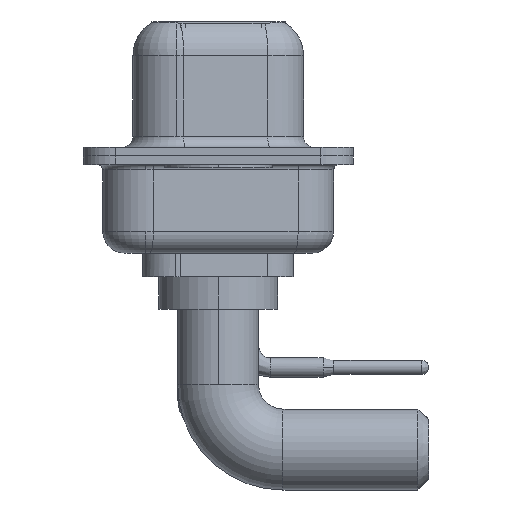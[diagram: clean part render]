
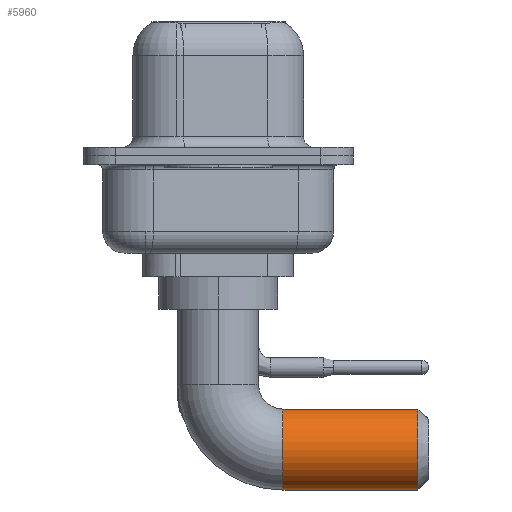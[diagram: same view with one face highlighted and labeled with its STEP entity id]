
A CAD part, left-side view. The second image highlights one B-rep face of the part: STEP entity #5960.
In plain terms, the highlighted cylindrical face has radius 1.875 mm (diameter 3.75 mm), a partial arc.
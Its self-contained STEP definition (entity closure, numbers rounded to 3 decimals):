
#13 = EDGE_CURVE ( 'NONE', #3064, #16424, #6679, .T. ) ;
#195 = DIRECTION ( 'NONE',  ( 0., -1., 0. ) ) ;
#295 = DIRECTION ( 'NONE',  ( -1., 0., 0. ) ) ;
#621 = DIRECTION ( 'NONE',  ( 0., -1., 0. ) ) ;
#923 = VERTEX_POINT ( 'NONE', #2142 ) ;
#1832 = LINE ( 'NONE', #17995, #5980 ) ;
#1844 = CARTESIAN_POINT ( 'NONE',  ( 0., -3., -8.375 ) ) ;
#2128 = ORIENTED_EDGE ( 'NONE', *, *, #6972, .T. ) ;
#2142 = CARTESIAN_POINT ( 'NONE',  ( 0., -3., -4.625 ) ) ;
#2319 = EDGE_CURVE ( 'NONE', #923, #16424, #1832, .T. ) ;
#2393 = ORIENTED_EDGE ( 'NONE', *, *, #2319, .F. ) ;
#3064 = VERTEX_POINT ( 'NONE', #11672 ) ;
#3971 = DIRECTION ( 'NONE',  ( 0., 0., -1. ) ) ;
#4563 = ORIENTED_EDGE ( 'NONE', *, *, #16297, .T. ) ;
#4697 = DIRECTION ( 'NONE',  ( 0., 0., -1. ) ) ;
#5217 = CARTESIAN_POINT ( 'NONE',  ( 0., -3., -8.375 ) ) ;
#5299 = CARTESIAN_POINT ( 'NONE',  ( 0., -3., -6.5 ) ) ;
#5551 = EDGE_LOOP ( 'NONE', ( #2393, #4563, #2128, #10373 ) ) ;
#5960 = ADVANCED_FACE ( 'NONE', ( #13280 ), #17560, .T. ) ;
#5980 = VECTOR ( 'NONE', #19631, 1000. ) ;
#6141 = AXIS2_PLACEMENT_3D ( 'NONE', #9312, #7980, #4697 ) ;
#6650 = CARTESIAN_POINT ( 'NONE',  ( 0., -3., -6.5 ) ) ;
#6679 = CIRCLE ( 'NONE', #6141, 1.875 ) ;
#6754 = VERTEX_POINT ( 'NONE', #1844 ) ;
#6972 = EDGE_CURVE ( 'NONE', #6754, #3064, #17808, .T. ) ;
#7980 = DIRECTION ( 'NONE',  ( 0., 1., 0. ) ) ;
#8620 = CIRCLE ( 'NONE', #19388, 1.875 ) ;
#9312 = CARTESIAN_POINT ( 'NONE',  ( 0., -9.25, -6.5 ) ) ;
#9823 = CARTESIAN_POINT ( 'NONE',  ( 0., -9.25, -4.625 ) ) ;
#10373 = ORIENTED_EDGE ( 'NONE', *, *, #13, .T. ) ;
#11672 = CARTESIAN_POINT ( 'NONE',  ( 0., -9.25, -8.375 ) ) ;
#11733 = DIRECTION ( 'NONE',  ( 0., -1., 0. ) ) ;
#13280 = FACE_OUTER_BOUND ( 'NONE', #5551, .T. ) ;
#15637 = AXIS2_PLACEMENT_3D ( 'NONE', #5299, #11733, #3971 ) ;
#16297 = EDGE_CURVE ( 'NONE', #923, #6754, #8620, .T. ) ;
#16424 = VERTEX_POINT ( 'NONE', #9823 ) ;
#16699 = VECTOR ( 'NONE', #621, 1000. ) ;
#17560 = CYLINDRICAL_SURFACE ( 'NONE', #15637, 1.875 ) ;
#17808 = LINE ( 'NONE', #5217, #16699 ) ;
#17995 = CARTESIAN_POINT ( 'NONE',  ( 0., -3., -4.625 ) ) ;
#19388 = AXIS2_PLACEMENT_3D ( 'NONE', #6650, #195, #295 ) ;
#19631 = DIRECTION ( 'NONE',  ( 0., -1., 0. ) ) ;
